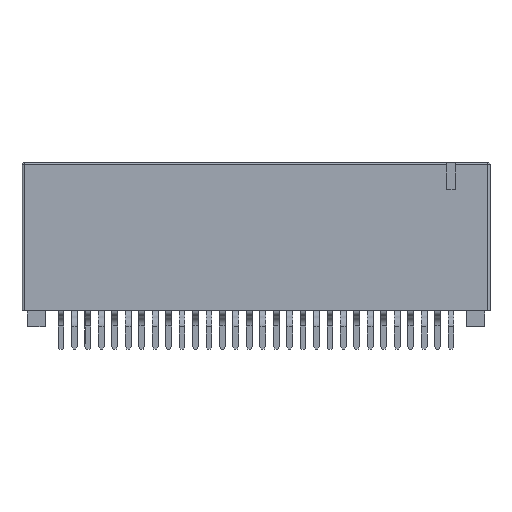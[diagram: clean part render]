
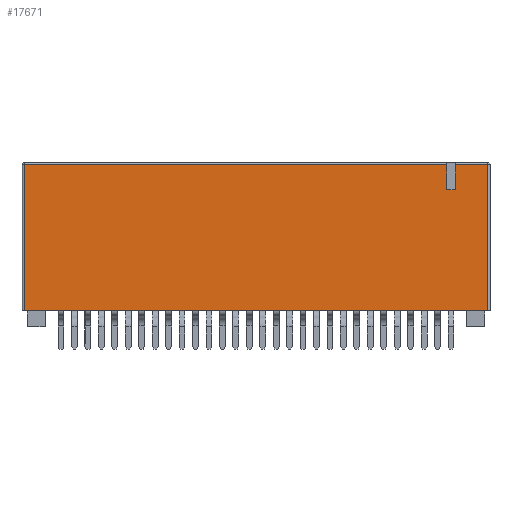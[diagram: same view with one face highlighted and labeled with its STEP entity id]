
A CAD part, top view. The second image highlights one B-rep face of the part: STEP entity #17671.
In plain terms, the highlighted planar face has unit normal (0, 0, 1).
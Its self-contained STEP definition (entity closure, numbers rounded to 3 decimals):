
#227 = CARTESIAN_POINT ( 'NONE',  ( 44., 1.5, 0. ) ) ;
#630 = DIRECTION ( 'NONE',  ( -1., 0., 0. ) ) ;
#824 = VERTEX_POINT ( 'NONE', #7766 ) ;
#846 = VECTOR ( 'NONE', #2728, 1000. ) ;
#1076 = CARTESIAN_POINT ( 'NONE',  ( 0.2, 15.3, 0. ) ) ;
#1367 = DIRECTION ( 'NONE',  ( 1., 0., 0. ) ) ;
#2338 = DIRECTION ( 'NONE',  ( 0., 0., -1. ) ) ;
#2402 = VECTOR ( 'NONE', #8269, 1000. ) ;
#2411 = EDGE_CURVE ( 'NONE', #3931, #20942, #4168, .T. ) ;
#2678 = DIRECTION ( 'NONE',  ( 0., 1., 0. ) ) ;
#2728 = DIRECTION ( 'NONE',  ( 0., 1., 0. ) ) ;
#3829 = CARTESIAN_POINT ( 'NONE',  ( 44.2, 1.5, 0. ) ) ;
#3844 = ORIENTED_EDGE ( 'NONE', *, *, #2411, .T. ) ;
#3931 = VERTEX_POINT ( 'NONE', #1076 ) ;
#4168 = LINE ( 'NONE', #16039, #15794 ) ;
#4268 = CARTESIAN_POINT ( 'NONE',  ( 0., 15.3, 0. ) ) ;
#4344 = LINE ( 'NONE', #20053, #20282 ) ;
#4368 = EDGE_CURVE ( 'NONE', #10158, #8063, #16912, .T. ) ;
#4665 = VECTOR ( 'NONE', #19295, 1000. ) ;
#5043 = VERTEX_POINT ( 'NONE', #11088 ) ;
#6219 = EDGE_CURVE ( 'NONE', #8063, #3931, #12909, .T. ) ;
#6463 = LINE ( 'NONE', #18186, #846 ) ;
#7766 = CARTESIAN_POINT ( 'NONE',  ( 40.905, 15.3, 0. ) ) ;
#7904 = EDGE_CURVE ( 'NONE', #5043, #824, #22650, .T. ) ;
#8063 = VERTEX_POINT ( 'NONE', #20964 ) ;
#8269 = DIRECTION ( 'NONE',  ( -1., 0., 0. ) ) ;
#9356 = LINE ( 'NONE', #15155, #21543 ) ;
#10158 = VERTEX_POINT ( 'NONE', #12796 ) ;
#11088 = CARTESIAN_POINT ( 'NONE',  ( 44., 15.3, 0. ) ) ;
#11192 = CARTESIAN_POINT ( 'NONE',  ( 40.905, 12.95, 0. ) ) ;
#11698 = VECTOR ( 'NONE', #16528, 1000. ) ;
#11729 = EDGE_LOOP ( 'NONE', ( #22540, #21047, #19095, #3844, #18937, #16062, #15484, #12815 ) ) ;
#11988 = VECTOR ( 'NONE', #630, 1000. ) ;
#12075 = EDGE_CURVE ( 'NONE', #24334, #20942, #25079, .T. ) ;
#12511 = EDGE_CURVE ( 'NONE', #10158, #19558, #9356, .T. ) ;
#12796 = CARTESIAN_POINT ( 'NONE',  ( 40.125, 12.95, 0. ) ) ;
#12815 = ORIENTED_EDGE ( 'NONE', *, *, #18959, .F. ) ;
#12909 = LINE ( 'NONE', #14450, #11988 ) ;
#14450 = CARTESIAN_POINT ( 'NONE',  ( 0., 15.3, 0. ) ) ;
#14458 = FACE_OUTER_BOUND ( 'NONE', #11729, .T. ) ;
#15155 = CARTESIAN_POINT ( 'NONE',  ( 40.125, 12.95, 0. ) ) ;
#15484 = ORIENTED_EDGE ( 'NONE', *, *, #7904, .T. ) ;
#15794 = VECTOR ( 'NONE', #23608, 1000. ) ;
#16039 = CARTESIAN_POINT ( 'NONE',  ( 0.2, 15.5, 0. ) ) ;
#16062 = ORIENTED_EDGE ( 'NONE', *, *, #21270, .T. ) ;
#16257 = DIRECTION ( 'NONE',  ( -1., 0., 0. ) ) ;
#16528 = DIRECTION ( 'NONE',  ( 0., 1., 0. ) ) ;
#16685 = AXIS2_PLACEMENT_3D ( 'NONE', #23948, #2338, #16257 ) ;
#16912 = LINE ( 'NONE', #24503, #11698 ) ;
#17671 = ADVANCED_FACE ( 'NONE', ( #14458 ), #22284, .F. ) ;
#18186 = CARTESIAN_POINT ( 'NONE',  ( 40.905, 12.95, 0. ) ) ;
#18799 = CARTESIAN_POINT ( 'NONE',  ( 0.2, 1.5, 0. ) ) ;
#18937 = ORIENTED_EDGE ( 'NONE', *, *, #12075, .F. ) ;
#18959 = EDGE_CURVE ( 'NONE', #19558, #824, #6463, .T. ) ;
#19095 = ORIENTED_EDGE ( 'NONE', *, *, #6219, .T. ) ;
#19295 = DIRECTION ( 'NONE',  ( -1., 0., 0. ) ) ;
#19558 = VERTEX_POINT ( 'NONE', #11192 ) ;
#20053 = CARTESIAN_POINT ( 'NONE',  ( 44., 15.5, 0. ) ) ;
#20282 = VECTOR ( 'NONE', #2678, 1000. ) ;
#20942 = VERTEX_POINT ( 'NONE', #18799 ) ;
#20964 = CARTESIAN_POINT ( 'NONE',  ( 40.125, 15.3, 0. ) ) ;
#21047 = ORIENTED_EDGE ( 'NONE', *, *, #4368, .T. ) ;
#21270 = EDGE_CURVE ( 'NONE', #24334, #5043, #4344, .T. ) ;
#21543 = VECTOR ( 'NONE', #1367, 1000. ) ;
#22284 = PLANE ( 'NONE',  #16685 ) ;
#22540 = ORIENTED_EDGE ( 'NONE', *, *, #12511, .F. ) ;
#22650 = LINE ( 'NONE', #4268, #2402 ) ;
#23608 = DIRECTION ( 'NONE',  ( 0., -1., 0. ) ) ;
#23948 = CARTESIAN_POINT ( 'NONE',  ( 0., 15.5, 0. ) ) ;
#24334 = VERTEX_POINT ( 'NONE', #227 ) ;
#24503 = CARTESIAN_POINT ( 'NONE',  ( 40.125, 12.95, 0. ) ) ;
#25079 = LINE ( 'NONE', #3829, #4665 ) ;
